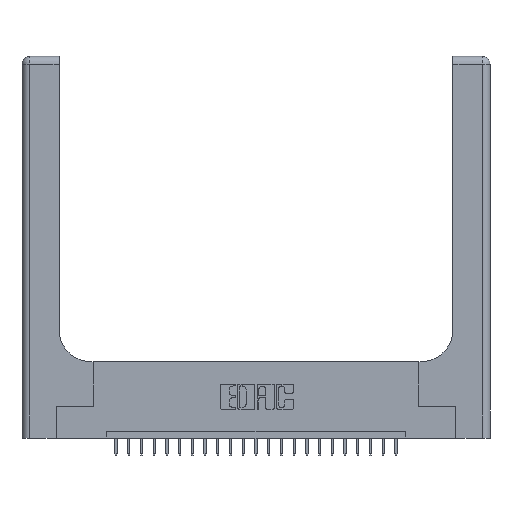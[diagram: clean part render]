
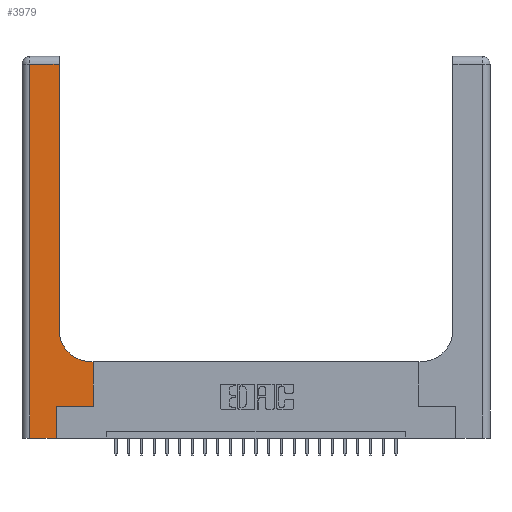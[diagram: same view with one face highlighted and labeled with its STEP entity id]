
A CAD part, top view. The second image highlights one B-rep face of the part: STEP entity #3979.
In plain terms, the highlighted planar face has unit normal (0, 0, 1).
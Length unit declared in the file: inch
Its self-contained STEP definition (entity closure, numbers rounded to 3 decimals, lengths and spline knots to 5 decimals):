
#54 = VERTEX_POINT ( 'NONE', #8663 ) ;
#1735 = DIRECTION ( 'NONE',  ( 0., 1., 0. ) ) ;
#1736 = VERTEX_POINT ( 'NONE', #8403 ) ;
#2157 = EDGE_CURVE ( 'NONE', #11282, #15762, #9262, .T. ) ;
#2326 = ORIENTED_EDGE ( 'NONE', *, *, #2157, .T. ) ;
#2782 = EDGE_CURVE ( 'NONE', #15799, #11994, #17166, .T. ) ;
#2969 = VECTOR ( 'NONE', #7335, 39.37008 ) ;
#3212 = EDGE_CURVE ( 'NONE', #11994, #54, #8813, .T. ) ;
#3279 = CARTESIAN_POINT ( 'NONE',  ( 0., 2.94, 0.37 ) ) ;
#3824 = CARTESIAN_POINT ( 'NONE',  ( 0.2915, 0.85, 0.37 ) ) ;
#3979 = ADVANCED_FACE ( 'NONE', ( #22528 ), #24417, .F. ) ;
#4481 = ORIENTED_EDGE ( 'NONE', *, *, #17684, .T. ) ;
#4558 = DIRECTION ( 'NONE',  ( -1., 0., 0. ) ) ;
#4886 = LINE ( 'NONE', #20718, #12744 ) ;
#4895 = CARTESIAN_POINT ( 'NONE',  ( 0.5585, 0.6, 0.37 ) ) ;
#5304 = CARTESIAN_POINT ( 'NONE',  ( 0.5585, 0.25, 0.37 ) ) ;
#6143 = CARTESIAN_POINT ( 'NONE',  ( 0.269, 0., 0.37 ) ) ;
#6785 = DIRECTION ( 'NONE',  ( 0., 0., -1. ) ) ;
#6844 = EDGE_CURVE ( 'NONE', #1736, #11395, #8938, .T. ) ;
#7057 = CARTESIAN_POINT ( 'NONE',  ( 0.2915, 3., 0.37 ) ) ;
#7114 = VECTOR ( 'NONE', #15173, 39.37008 ) ;
#7335 = DIRECTION ( 'NONE',  ( 1., 0., 0. ) ) ;
#7752 = ORIENTED_EDGE ( 'NONE', *, *, #13958, .T. ) ;
#8216 = LINE ( 'NONE', #6143, #22410 ) ;
#8403 = CARTESIAN_POINT ( 'NONE',  ( 0.06, 0., 0.37 ) ) ;
#8663 = CARTESIAN_POINT ( 'NONE',  ( 0.5415, 0.6, 0.37 ) ) ;
#8813 = LINE ( 'NONE', #14670, #12704 ) ;
#8840 = CARTESIAN_POINT ( 'NONE',  ( 0.06, 2.94, 0.37 ) ) ;
#8938 = LINE ( 'NONE', #9187, #7114 ) ;
#9187 = CARTESIAN_POINT ( 'NONE',  ( 0., 0., 0.37 ) ) ;
#9262 = LINE ( 'NONE', #7057, #15111 ) ;
#9812 = CARTESIAN_POINT ( 'NONE',  ( 0.5585, 0.25, 0.37 ) ) ;
#9898 = ORIENTED_EDGE ( 'NONE', *, *, #19874, .T. ) ;
#9947 = CARTESIAN_POINT ( 'NONE',  ( 0.269, 0.25, 0.37 ) ) ;
#10400 = ORIENTED_EDGE ( 'NONE', *, *, #2782, .T. ) ;
#10808 = DIRECTION ( 'NONE',  ( 0., -1., 0. ) ) ;
#11282 = VERTEX_POINT ( 'NONE', #3824 ) ;
#11395 = VERTEX_POINT ( 'NONE', #21912 ) ;
#11944 = AXIS2_PLACEMENT_3D ( 'NONE', #20376, #20637, #4558 ) ;
#11994 = VERTEX_POINT ( 'NONE', #4895 ) ;
#12271 = EDGE_CURVE ( 'NONE', #11395, #20768, #8216, .T. ) ;
#12602 = VERTEX_POINT ( 'NONE', #8840 ) ;
#12704 = VECTOR ( 'NONE', #14426, 39.37008 ) ;
#12744 = VECTOR ( 'NONE', #10808, 39.37008 ) ;
#13145 = ORIENTED_EDGE ( 'NONE', *, *, #17488, .T. ) ;
#13744 = CARTESIAN_POINT ( 'NONE',  ( 0.2915, 2.94, 0.37 ) ) ;
#13958 = EDGE_CURVE ( 'NONE', #15762, #12602, #20759, .T. ) ;
#14426 = DIRECTION ( 'NONE',  ( -1., 0., 0. ) ) ;
#14605 = DIRECTION ( 'NONE',  ( 1., 0., 0. ) ) ;
#14670 = CARTESIAN_POINT ( 'NONE',  ( 0.2915, 0.6, 0.37 ) ) ;
#14997 = ORIENTED_EDGE ( 'NONE', *, *, #6844, .T. ) ;
#15111 = VECTOR ( 'NONE', #17021, 39.37008 ) ;
#15173 = DIRECTION ( 'NONE',  ( 1., 0., 0. ) ) ;
#15762 = VERTEX_POINT ( 'NONE', #13744 ) ;
#15799 = VERTEX_POINT ( 'NONE', #9812 ) ;
#17021 = DIRECTION ( 'NONE',  ( 0., 1., 0. ) ) ;
#17166 = LINE ( 'NONE', #5304, #22440 ) ;
#17488 = EDGE_CURVE ( 'NONE', #12602, #1736, #4886, .T. ) ;
#17684 = EDGE_CURVE ( 'NONE', #54, #11282, #20890, .T. ) ;
#18839 = DIRECTION ( 'NONE',  ( -1., 0., 0. ) ) ;
#19096 = VECTOR ( 'NONE', #18839, 39.37008 ) ;
#19163 = LINE ( 'NONE', #24753, #2969 ) ;
#19491 = ORIENTED_EDGE ( 'NONE', *, *, #12271, .T. ) ;
#19874 = EDGE_CURVE ( 'NONE', #20768, #15799, #19163, .T. ) ;
#20063 = DIRECTION ( 'NONE',  ( 0., 1., 0. ) ) ;
#20376 = CARTESIAN_POINT ( 'NONE',  ( 0., 3., 0.37 ) ) ;
#20637 = DIRECTION ( 'NONE',  ( 0., 0., -1. ) ) ;
#20718 = CARTESIAN_POINT ( 'NONE',  ( 0.06, 3., 0.37 ) ) ;
#20759 = LINE ( 'NONE', #3279, #19096 ) ;
#20768 = VERTEX_POINT ( 'NONE', #9947 ) ;
#20890 = CIRCLE ( 'NONE', #22069, 0.25 ) ;
#21912 = CARTESIAN_POINT ( 'NONE',  ( 0.269, 0., 0.37 ) ) ;
#22069 = AXIS2_PLACEMENT_3D ( 'NONE', #24221, #6785, #14605 ) ;
#22159 = EDGE_LOOP ( 'NONE', ( #2326, #7752, #13145, #14997, #19491, #9898, #10400, #22723, #4481 ) ) ;
#22410 = VECTOR ( 'NONE', #20063, 39.37008 ) ;
#22440 = VECTOR ( 'NONE', #1735, 39.37008 ) ;
#22528 = FACE_OUTER_BOUND ( 'NONE', #22159, .T. ) ;
#22723 = ORIENTED_EDGE ( 'NONE', *, *, #3212, .T. ) ;
#24221 = CARTESIAN_POINT ( 'NONE',  ( 0.5415, 0.85, 0.37 ) ) ;
#24417 = PLANE ( 'NONE',  #11944 ) ;
#24753 = CARTESIAN_POINT ( 'NONE',  ( 0.269, 0.25, 0.37 ) ) ;
